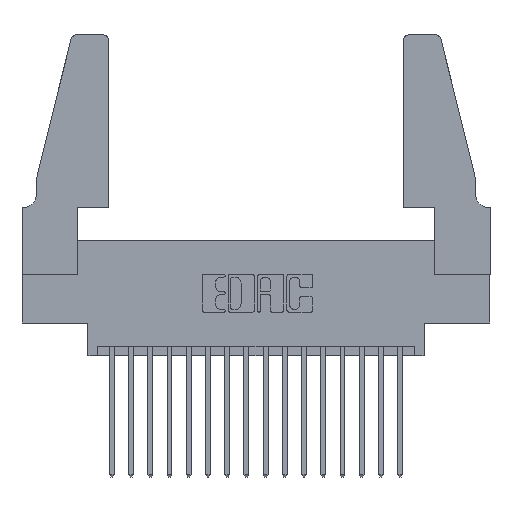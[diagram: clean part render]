
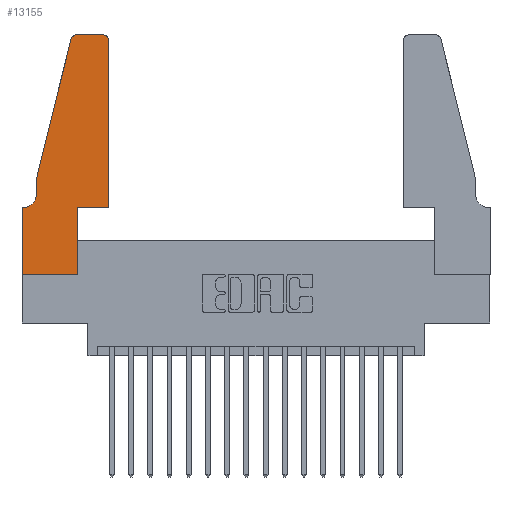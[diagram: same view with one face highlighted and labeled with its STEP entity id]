
A CAD part, top view. The second image highlights one B-rep face of the part: STEP entity #13155.
In plain terms, the highlighted planar face has unit normal (0, 0, 1).
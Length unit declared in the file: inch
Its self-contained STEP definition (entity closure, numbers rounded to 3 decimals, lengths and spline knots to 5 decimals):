
#8 = VERTEX_POINT ( 'NONE', #10472 ) ;
#425 = DIRECTION ( 'NONE',  ( 0., -1., 0. ) ) ;
#614 = AXIS2_PLACEMENT_3D ( 'NONE', #10613, #14865, #9237 ) ;
#1093 = FACE_OUTER_BOUND ( 'NONE', #12345, .T. ) ;
#1152 = VERTEX_POINT ( 'NONE', #8539 ) ;
#1380 = LINE ( 'NONE', #3245, #4897 ) ;
#1443 = AXIS2_PLACEMENT_3D ( 'NONE', #8981, #6079, #1461 ) ;
#1461 = DIRECTION ( 'NONE',  ( 1., 0., 0. ) ) ;
#1494 = CARTESIAN_POINT ( 'NONE',  ( 0., 0., 0.37 ) ) ;
#1554 = DIRECTION ( 'NONE',  ( 1., 0., 0. ) ) ;
#1564 = ORIENTED_EDGE ( 'NONE', *, *, #9995, .T. ) ;
#1752 = VECTOR ( 'NONE', #13617, 39.37008 ) ;
#1961 = EDGE_CURVE ( 'NONE', #8635, #8853, #3476, .T. ) ;
#1980 = DIRECTION ( 'NONE',  ( -0.239, -0.971, 0. ) ) ;
#2339 = ORIENTED_EDGE ( 'NONE', *, *, #5489, .T. ) ;
#2483 = VECTOR ( 'NONE', #4733, 39.37008 ) ;
#3245 = CARTESIAN_POINT ( 'NONE',  ( 0.2865, 0.35, 0.37 ) ) ;
#3476 = CIRCLE ( 'NONE', #1443, 0.03 ) ;
#3485 = CARTESIAN_POINT ( 'NONE',  ( 0.4205, 1.25, 0.37 ) ) ;
#3530 = CARTESIAN_POINT ( 'NONE',  ( 0.25487, 1.22718, 0.37 ) ) ;
#3541 = DIRECTION ( 'NONE',  ( 1., 0., 0. ) ) ;
#3628 = LINE ( 'NONE', #1494, #16708 ) ;
#4233 = LINE ( 'NONE', #10874, #2483 ) ;
#4683 = AXIS2_PLACEMENT_3D ( 'NONE', #13427, #12028, #3541 ) ;
#4733 = DIRECTION ( 'NONE',  ( 0., -1., 0. ) ) ;
#4754 = DIRECTION ( 'NONE',  ( 0., 0., -1. ) ) ;
#4788 = CARTESIAN_POINT ( 'NONE',  ( 0.0755, 0.5, 0.37 ) ) ;
#4897 = VECTOR ( 'NONE', #16054, 39.37008 ) ;
#4983 = LINE ( 'NONE', #14215, #16993 ) ;
#5079 = LINE ( 'NONE', #5417, #8392 ) ;
#5250 = CARTESIAN_POINT ( 'NONE',  ( 0.2605, 1.25, 0.37 ) ) ;
#5417 = CARTESIAN_POINT ( 'NONE',  ( 0.0755, 0.35, 0.37 ) ) ;
#5489 = EDGE_CURVE ( 'NONE', #8853, #18380, #4983, .T. ) ;
#5529 = ORIENTED_EDGE ( 'NONE', *, *, #14034, .T. ) ;
#5894 = EDGE_CURVE ( 'NONE', #13640, #1152, #7832, .T. ) ;
#6079 = DIRECTION ( 'NONE',  ( 0., 0., 1. ) ) ;
#6235 = CARTESIAN_POINT ( 'NONE',  ( 0.284, 1.25, 0.37 ) ) ;
#6242 = ORIENTED_EDGE ( 'NONE', *, *, #11295, .T. ) ;
#6625 = EDGE_CURVE ( 'NONE', #8, #9714, #3628, .T. ) ;
#6663 = ORIENTED_EDGE ( 'NONE', *, *, #12056, .T. ) ;
#7269 = VERTEX_POINT ( 'NONE', #13624 ) ;
#7832 = LINE ( 'NONE', #13723, #13612 ) ;
#8196 = DIRECTION ( 'NONE',  ( -1., 0., 0. ) ) ;
#8221 = EDGE_CURVE ( 'NONE', #14983, #14660, #15963, .T. ) ;
#8230 = VECTOR ( 'NONE', #15991, 39.37008 ) ;
#8274 = ORIENTED_EDGE ( 'NONE', *, *, #11394, .T. ) ;
#8392 = VECTOR ( 'NONE', #8196, 39.37008 ) ;
#8456 = EDGE_CURVE ( 'NONE', #12636, #8635, #11765, .T. ) ;
#8539 = CARTESIAN_POINT ( 'NONE',  ( 0.4505, 0.35, 0.37 ) ) ;
#8586 = AXIS2_PLACEMENT_3D ( 'NONE', #8949, #4754, #17475 ) ;
#8635 = VERTEX_POINT ( 'NONE', #6235 ) ;
#8853 = VERTEX_POINT ( 'NONE', #3530 ) ;
#8949 = CARTESIAN_POINT ( 'NONE',  ( 0.0055, 0.42, 0.37 ) ) ;
#8981 = CARTESIAN_POINT ( 'NONE',  ( 0.284, 1.22, 0.37 ) ) ;
#9124 = CARTESIAN_POINT ( 'NONE',  ( 0.2865, 0.35, 0.37 ) ) ;
#9237 = DIRECTION ( 'NONE',  ( 1., 0., 0. ) ) ;
#9714 = VERTEX_POINT ( 'NONE', #18218 ) ;
#9995 = EDGE_CURVE ( 'NONE', #7269, #12636, #18137, .T. ) ;
#10142 = LINE ( 'NONE', #14223, #12386 ) ;
#10234 = CARTESIAN_POINT ( 'NONE',  ( 0.4505, 0.35, 0.37 ) ) ;
#10472 = CARTESIAN_POINT ( 'NONE',  ( 0., 0., 0.37 ) ) ;
#10613 = CARTESIAN_POINT ( 'NONE',  ( 0.4205, 1.22, 0.37 ) ) ;
#10634 = DIRECTION ( 'NONE',  ( 1., 0., 0. ) ) ;
#10874 = CARTESIAN_POINT ( 'NONE',  ( 0.0755, 0.5, 0.37 ) ) ;
#11276 = ORIENTED_EDGE ( 'NONE', *, *, #6625, .T. ) ;
#11295 = EDGE_CURVE ( 'NONE', #1152, #7269, #16694, .T. ) ;
#11394 = EDGE_CURVE ( 'NONE', #9714, #13640, #1380, .T. ) ;
#11765 = LINE ( 'NONE', #5250, #1752 ) ;
#11973 = PLANE ( 'NONE',  #4683 ) ;
#12028 = DIRECTION ( 'NONE',  ( 0., 0., 1. ) ) ;
#12056 = EDGE_CURVE ( 'NONE', #18380, #14983, #4233, .T. ) ;
#12072 = VERTEX_POINT ( 'NONE', #14831 ) ;
#12196 = ORIENTED_EDGE ( 'NONE', *, *, #5894, .T. ) ;
#12345 = EDGE_LOOP ( 'NONE', ( #14016, #13354, #2339, #6663, #13495, #17300, #5529, #11276, #8274, #12196, #6242, #1564 ) ) ;
#12386 = VECTOR ( 'NONE', #425, 39.37008 ) ;
#12636 = VERTEX_POINT ( 'NONE', #3485 ) ;
#12727 = EDGE_CURVE ( 'NONE', #14660, #12072, #5079, .T. ) ;
#13155 = ADVANCED_FACE ( 'NONE', ( #1093 ), #11973, .T. ) ;
#13354 = ORIENTED_EDGE ( 'NONE', *, *, #1961, .T. ) ;
#13427 = CARTESIAN_POINT ( 'NONE',  ( 0., 0.35, 0.37 ) ) ;
#13495 = ORIENTED_EDGE ( 'NONE', *, *, #8221, .T. ) ;
#13612 = VECTOR ( 'NONE', #10634, 39.37008 ) ;
#13617 = DIRECTION ( 'NONE',  ( -1., 0., 0. ) ) ;
#13624 = CARTESIAN_POINT ( 'NONE',  ( 0.4505, 1.22, 0.37 ) ) ;
#13640 = VERTEX_POINT ( 'NONE', #9124 ) ;
#13723 = CARTESIAN_POINT ( 'NONE',  ( 0.4505, 0.35, 0.37 ) ) ;
#14016 = ORIENTED_EDGE ( 'NONE', *, *, #8456, .T. ) ;
#14034 = EDGE_CURVE ( 'NONE', #12072, #8, #10142, .T. ) ;
#14215 = CARTESIAN_POINT ( 'NONE',  ( 0.0755, 0.5, 0.37 ) ) ;
#14223 = CARTESIAN_POINT ( 'NONE',  ( 0., 0., 0.37 ) ) ;
#14626 = CARTESIAN_POINT ( 'NONE',  ( 0.0755, 0.42, 0.37 ) ) ;
#14660 = VERTEX_POINT ( 'NONE', #15717 ) ;
#14831 = CARTESIAN_POINT ( 'NONE',  ( 0., 0.35, 0.37 ) ) ;
#14865 = DIRECTION ( 'NONE',  ( 0., 0., 1. ) ) ;
#14983 = VERTEX_POINT ( 'NONE', #14626 ) ;
#15717 = CARTESIAN_POINT ( 'NONE',  ( 0.0055, 0.35, 0.37 ) ) ;
#15963 = CIRCLE ( 'NONE', #8586, 0.07 ) ;
#15991 = DIRECTION ( 'NONE',  ( 0., 1., 0. ) ) ;
#16054 = DIRECTION ( 'NONE',  ( 0., 1., 0. ) ) ;
#16694 = LINE ( 'NONE', #10234, #8230 ) ;
#16708 = VECTOR ( 'NONE', #1554, 39.37008 ) ;
#16993 = VECTOR ( 'NONE', #1980, 39.37008 ) ;
#17300 = ORIENTED_EDGE ( 'NONE', *, *, #12727, .T. ) ;
#17475 = DIRECTION ( 'NONE',  ( -1., 0., 0. ) ) ;
#18137 = CIRCLE ( 'NONE', #614, 0.03 ) ;
#18218 = CARTESIAN_POINT ( 'NONE',  ( 0.2865, 0., 0.37 ) ) ;
#18380 = VERTEX_POINT ( 'NONE', #4788 ) ;
